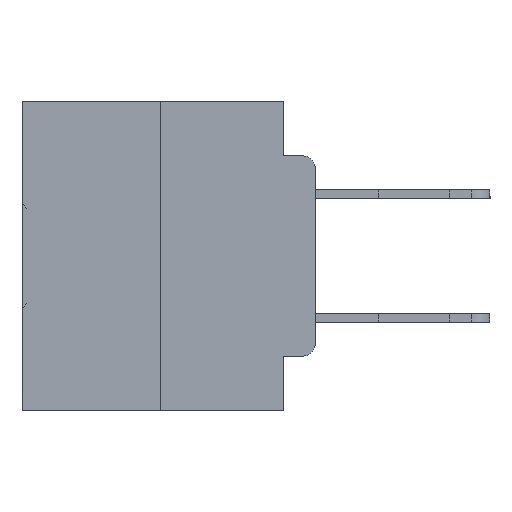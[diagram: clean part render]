
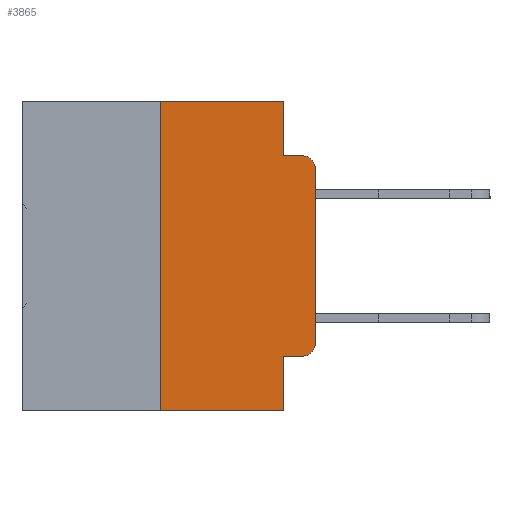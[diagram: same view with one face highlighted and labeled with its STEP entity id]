
A CAD part, left-side view. The second image highlights one B-rep face of the part: STEP entity #3865.
In plain terms, the highlighted planar face has unit normal (-1, 0, 0).
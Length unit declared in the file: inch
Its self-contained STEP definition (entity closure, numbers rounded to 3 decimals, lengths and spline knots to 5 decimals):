
#83 = EDGE_CURVE ( 'NONE', #19148, #894, #30258, .T. ) ;
#337 = VERTEX_POINT ( 'NONE', #6015 ) ;
#560 = EDGE_CURVE ( 'NONE', #29171, #14264, #30224, .T. ) ;
#856 = DIRECTION ( 'NONE',  ( 0., 0., -1. ) ) ;
#894 = VERTEX_POINT ( 'NONE', #25979 ) ;
#1930 = VERTEX_POINT ( 'NONE', #25326 ) ;
#2167 = VERTEX_POINT ( 'NONE', #18320 ) ;
#2184 = CARTESIAN_POINT ( 'NONE',  ( 0., 0.02, -0.3915 ) ) ;
#2447 = CARTESIAN_POINT ( 'NONE',  ( 0., 0.051, -0.4115 ) ) ;
#2530 = VERTEX_POINT ( 'NONE', #9616 ) ;
#2618 = VECTOR ( 'NONE', #33088, 39.37008 ) ;
#3042 = VECTOR ( 'NONE', #33902, 39.37008 ) ;
#3066 = ORIENTED_EDGE ( 'NONE', *, *, #83, .T. ) ;
#3488 = LINE ( 'NONE', #25094, #2618 ) ;
#3865 = ADVANCED_FACE ( 'NONE', ( #18853 ), #6634, .F. ) ;
#4134 = VERTEX_POINT ( 'NONE', #10293 ) ;
#4188 = ORIENTED_EDGE ( 'NONE', *, *, #27729, .T. ) ;
#4726 = LINE ( 'NONE', #31479, #25405 ) ;
#5035 = DIRECTION ( 'NONE',  ( 0., 0., -1. ) ) ;
#6015 = CARTESIAN_POINT ( 'NONE',  ( 0., 0., -0.1085 ) ) ;
#6046 = VECTOR ( 'NONE', #856, 39.37008 ) ;
#6464 = ORIENTED_EDGE ( 'NONE', *, *, #27121, .F. ) ;
#6540 = DIRECTION ( 'NONE',  ( 0., 0., 1. ) ) ;
#6552 = EDGE_CURVE ( 'NONE', #4134, #31099, #3488, .T. ) ;
#6634 = PLANE ( 'NONE',  #19397 ) ;
#6909 = LINE ( 'NONE', #20044, #6046 ) ;
#6918 = CARTESIAN_POINT ( 'NONE',  ( 0., 0.02, -0.1085 ) ) ;
#7697 = ORIENTED_EDGE ( 'NONE', *, *, #32415, .F. ) ;
#8018 = CARTESIAN_POINT ( 'NONE',  ( 0., 0.051, -0.4115 ) ) ;
#8204 = ORIENTED_EDGE ( 'NONE', *, *, #29985, .F. ) ;
#9616 = CARTESIAN_POINT ( 'NONE',  ( 0., 0., -0.3915 ) ) ;
#9635 = EDGE_CURVE ( 'NONE', #337, #2167, #21141, .T. ) ;
#9674 = DIRECTION ( 'NONE',  ( 0., 0., -1. ) ) ;
#10080 = CARTESIAN_POINT ( 'NONE',  ( 0., 0.473, 0. ) ) ;
#10293 = CARTESIAN_POINT ( 'NONE',  ( 0., 0.051, 0. ) ) ;
#11812 = VECTOR ( 'NONE', #32612, 39.37008 ) ;
#12055 = EDGE_CURVE ( 'NONE', #894, #2530, #17725, .T. ) ;
#13123 = CARTESIAN_POINT ( 'NONE',  ( 0., 0.25, -0.5 ) ) ;
#13838 = EDGE_CURVE ( 'NONE', #31099, #2167, #24662, .T. ) ;
#14021 = CARTESIAN_POINT ( 'NONE',  ( 0., 0.473, 0. ) ) ;
#14264 = VERTEX_POINT ( 'NONE', #30497 ) ;
#15562 = DIRECTION ( 'NONE',  ( 0., 0., 1. ) ) ;
#17470 = ORIENTED_EDGE ( 'NONE', *, *, #6552, .F. ) ;
#17725 = CIRCLE ( 'NONE', #27587, 0.02 ) ;
#17908 = LINE ( 'NONE', #33221, #31196 ) ;
#18320 = CARTESIAN_POINT ( 'NONE',  ( 0., 0.02, -0.0885 ) ) ;
#18853 = FACE_OUTER_BOUND ( 'NONE', #28113, .T. ) ;
#19148 = VERTEX_POINT ( 'NONE', #8018 ) ;
#19397 = AXIS2_PLACEMENT_3D ( 'NONE', #10080, #22929, #25427 ) ;
#20044 = CARTESIAN_POINT ( 'NONE',  ( 0., 0.051, 0. ) ) ;
#21141 = CIRCLE ( 'NONE', #29325, 0.02 ) ;
#21258 = DIRECTION ( 'NONE',  ( -1., 0., 0. ) ) ;
#21506 = DIRECTION ( 'NONE',  ( 0., -1., 0. ) ) ;
#22033 = DIRECTION ( 'NONE',  ( 0., -1., 0. ) ) ;
#22929 = DIRECTION ( 'NONE',  ( 1., 0., 0. ) ) ;
#23176 = VECTOR ( 'NONE', #22033, 39.37008 ) ;
#23209 = VECTOR ( 'NONE', #21506, 39.37008 ) ;
#23879 = ORIENTED_EDGE ( 'NONE', *, *, #13838, .F. ) ;
#23956 = ORIENTED_EDGE ( 'NONE', *, *, #560, .T. ) ;
#24408 = ORIENTED_EDGE ( 'NONE', *, *, #12055, .T. ) ;
#24662 = LINE ( 'NONE', #31265, #3042 ) ;
#25094 = CARTESIAN_POINT ( 'NONE',  ( 0., 0.051, 0. ) ) ;
#25326 = CARTESIAN_POINT ( 'NONE',  ( 0., 0.25, 0. ) ) ;
#25405 = VECTOR ( 'NONE', #15562, 39.37008 ) ;
#25427 = DIRECTION ( 'NONE',  ( 0., 0., -1. ) ) ;
#25693 = DIRECTION ( 'NONE',  ( -1., 0., 0. ) ) ;
#25979 = CARTESIAN_POINT ( 'NONE',  ( 0., 0.02, -0.4115 ) ) ;
#26627 = ORIENTED_EDGE ( 'NONE', *, *, #9635, .T. ) ;
#27121 = EDGE_CURVE ( 'NONE', #19148, #14264, #6909, .T. ) ;
#27587 = AXIS2_PLACEMENT_3D ( 'NONE', #2184, #21258, #5035 ) ;
#27729 = EDGE_CURVE ( 'NONE', #2530, #337, #17908, .T. ) ;
#28113 = EDGE_LOOP ( 'NONE', ( #4188, #26627, #23879, #17470, #8204, #7697, #23956, #6464, #3066, #24408 ) ) ;
#29126 = CARTESIAN_POINT ( 'NONE',  ( 0., 0.473, -0.5 ) ) ;
#29171 = VERTEX_POINT ( 'NONE', #13123 ) ;
#29185 = CARTESIAN_POINT ( 'NONE',  ( 0., 0.051, -0.0885 ) ) ;
#29325 = AXIS2_PLACEMENT_3D ( 'NONE', #6918, #25693, #9674 ) ;
#29985 = EDGE_CURVE ( 'NONE', #1930, #4134, #32233, .T. ) ;
#30224 = LINE ( 'NONE', #29126, #23176 ) ;
#30258 = LINE ( 'NONE', #2447, #23209 ) ;
#30497 = CARTESIAN_POINT ( 'NONE',  ( 0., 0.051, -0.5 ) ) ;
#31099 = VERTEX_POINT ( 'NONE', #29185 ) ;
#31196 = VECTOR ( 'NONE', #6540, 39.37008 ) ;
#31265 = CARTESIAN_POINT ( 'NONE',  ( 0., 0.051, -0.0885 ) ) ;
#31479 = CARTESIAN_POINT ( 'NONE',  ( 0., 0.25, 0. ) ) ;
#32233 = LINE ( 'NONE', #14021, #11812 ) ;
#32415 = EDGE_CURVE ( 'NONE', #29171, #1930, #4726, .T. ) ;
#32612 = DIRECTION ( 'NONE',  ( 0., -1., 0. ) ) ;
#33088 = DIRECTION ( 'NONE',  ( 0., 0., -1. ) ) ;
#33221 = CARTESIAN_POINT ( 'NONE',  ( 0., 0., 0. ) ) ;
#33902 = DIRECTION ( 'NONE',  ( 0., -1., 0. ) ) ;
